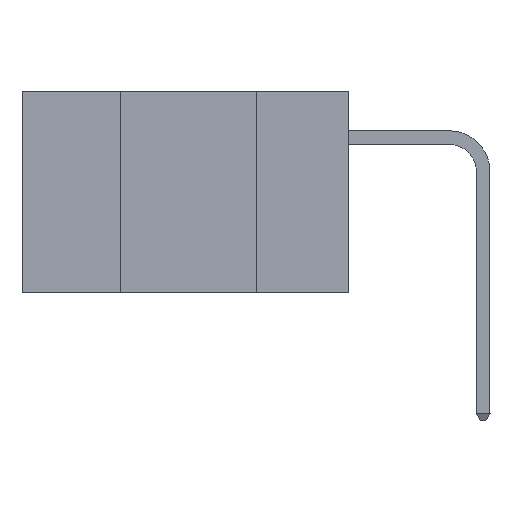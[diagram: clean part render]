
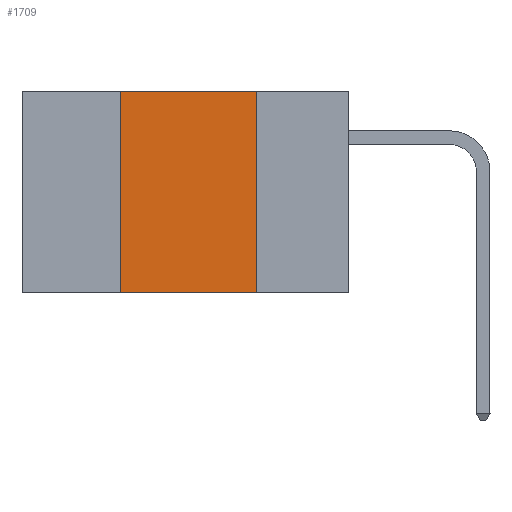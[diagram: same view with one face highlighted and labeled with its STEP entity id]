
A CAD part, left-side view. The second image highlights one B-rep face of the part: STEP entity #1709.
In plain terms, the highlighted planar face has unit normal (-1, 0, 0).
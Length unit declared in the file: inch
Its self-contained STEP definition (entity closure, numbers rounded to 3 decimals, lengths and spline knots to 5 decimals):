
#538 = DIRECTION ( 'NONE',  ( 1., 0., 0. ) ) ;
#547 = AXIS2_PLACEMENT_3D ( 'NONE', #16041, #538, #9908 ) ;
#686 = LINE ( 'NONE', #2092, #11472 ) ;
#916 = ORIENTED_EDGE ( 'NONE', *, *, #7298, .F. ) ;
#1274 = EDGE_CURVE ( 'NONE', #2101, #1681, #686, .T. ) ;
#1443 = CARTESIAN_POINT ( 'NONE',  ( 0., 0.17, 0. ) ) ;
#1681 = VERTEX_POINT ( 'NONE', #15838 ) ;
#1709 = ADVANCED_FACE ( 'NONE', ( #2040 ), #3765, .F. ) ;
#2040 = FACE_OUTER_BOUND ( 'NONE', #9637, .T. ) ;
#2092 = CARTESIAN_POINT ( 'NONE',  ( 0., 0.42, 0. ) ) ;
#2101 = VERTEX_POINT ( 'NONE', #14199 ) ;
#2482 = VECTOR ( 'NONE', #15417, 39.37008 ) ;
#2538 = VECTOR ( 'NONE', #15769, 39.37008 ) ;
#3139 = LINE ( 'NONE', #9284, #2482 ) ;
#3596 = CARTESIAN_POINT ( 'NONE',  ( 0., 0.6, -0.37 ) ) ;
#3765 = PLANE ( 'NONE',  #547 ) ;
#4606 = LINE ( 'NONE', #13769, #13407 ) ;
#4731 = VERTEX_POINT ( 'NONE', #1443 ) ;
#5135 = DIRECTION ( 'NONE',  ( 0., 0., 1. ) ) ;
#6309 = CARTESIAN_POINT ( 'NONE',  ( 0., 0.17, -0.37 ) ) ;
#6718 = LINE ( 'NONE', #3596, #2538 ) ;
#7298 = EDGE_CURVE ( 'NONE', #1681, #4731, #3139, .T. ) ;
#9284 = CARTESIAN_POINT ( 'NONE',  ( 0., 0.6, 0. ) ) ;
#9329 = VERTEX_POINT ( 'NONE', #6309 ) ;
#9498 = EDGE_CURVE ( 'NONE', #2101, #9329, #6718, .T. ) ;
#9637 = EDGE_LOOP ( 'NONE', ( #11882, #916, #13022, #18815 ) ) ;
#9908 = DIRECTION ( 'NONE',  ( 0., 0., -1. ) ) ;
#11472 = VECTOR ( 'NONE', #5135, 39.37008 ) ;
#11881 = DIRECTION ( 'NONE',  ( 0., 0., -1. ) ) ;
#11882 = ORIENTED_EDGE ( 'NONE', *, *, #19370, .F. ) ;
#13022 = ORIENTED_EDGE ( 'NONE', *, *, #1274, .F. ) ;
#13407 = VECTOR ( 'NONE', #11881, 39.37008 ) ;
#13769 = CARTESIAN_POINT ( 'NONE',  ( 0., 0.17, 0. ) ) ;
#14199 = CARTESIAN_POINT ( 'NONE',  ( 0., 0.42, -0.37 ) ) ;
#15417 = DIRECTION ( 'NONE',  ( 0., -1., 0. ) ) ;
#15769 = DIRECTION ( 'NONE',  ( 0., -1., 0. ) ) ;
#15838 = CARTESIAN_POINT ( 'NONE',  ( 0., 0.42, 0. ) ) ;
#16041 = CARTESIAN_POINT ( 'NONE',  ( 0., 0.6, 0. ) ) ;
#18815 = ORIENTED_EDGE ( 'NONE', *, *, #9498, .T. ) ;
#19370 = EDGE_CURVE ( 'NONE', #4731, #9329, #4606, .T. ) ;
